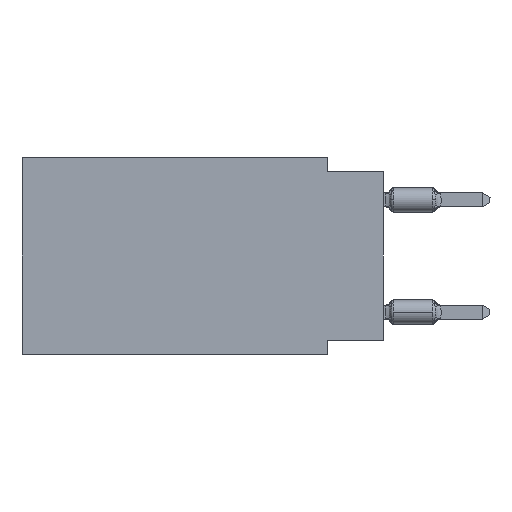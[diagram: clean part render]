
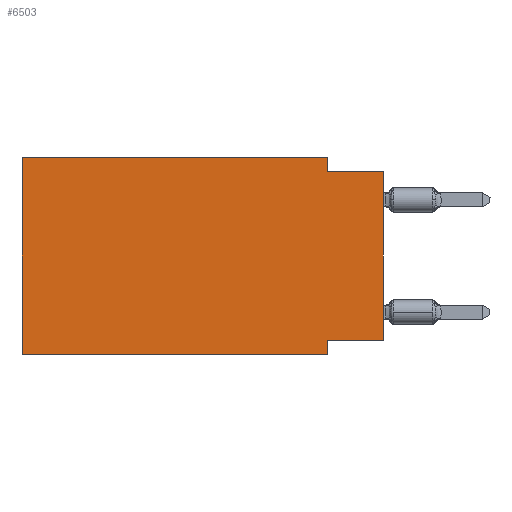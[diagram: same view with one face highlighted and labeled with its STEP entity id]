
A CAD part, left-side view. The second image highlights one B-rep face of the part: STEP entity #6503.
In plain terms, the highlighted planar face has unit normal (-1, 0, 0).
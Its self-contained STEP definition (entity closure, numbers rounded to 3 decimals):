
#836 = VECTOR ( 'NONE', #21411, 1000. ) ;
#2006 = DIRECTION ( 'NONE',  ( 0., -1., 0. ) ) ;
#2453 = CARTESIAN_POINT ( 'NONE',  ( 0., 0., -8.255 ) ) ;
#2573 = VERTEX_POINT ( 'NONE', #9083 ) ;
#2668 = ORIENTED_EDGE ( 'NONE', *, *, #27510, .F. ) ;
#3860 = VERTEX_POINT ( 'NONE', #21286 ) ;
#4321 = CARTESIAN_POINT ( 'NONE',  ( 0., 2.54, -0.635 ) ) ;
#4750 = CARTESIAN_POINT ( 'NONE',  ( 0., 2.54, -8.89 ) ) ;
#4767 = CARTESIAN_POINT ( 'NONE',  ( 0., 16.383, -8.89 ) ) ;
#6503 = ADVANCED_FACE ( 'NONE', ( #11510 ), #27806, .F. ) ;
#7463 = ORIENTED_EDGE ( 'NONE', *, *, #36338, .F. ) ;
#7663 = ORIENTED_EDGE ( 'NONE', *, *, #8486, .F. ) ;
#7884 = LINE ( 'NONE', #18130, #19427 ) ;
#8181 = LINE ( 'NONE', #14864, #32809 ) ;
#8486 = EDGE_CURVE ( 'NONE', #2573, #15020, #36292, .T. ) ;
#9083 = CARTESIAN_POINT ( 'NONE',  ( 0., 2.54, 0. ) ) ;
#10034 = EDGE_CURVE ( 'NONE', #3860, #40773, #40194, .T. ) ;
#10100 = VECTOR ( 'NONE', #2006, 1000. ) ;
#11232 = EDGE_LOOP ( 'NONE', ( #31197, #7463, #7663, #2668, #27136, #36452, #40490, #27331 ) ) ;
#11510 = FACE_OUTER_BOUND ( 'NONE', #11232, .T. ) ;
#11722 = CARTESIAN_POINT ( 'NONE',  ( 0., 16.383, 0. ) ) ;
#11844 = DIRECTION ( 'NONE',  ( 0., 0., 1. ) ) ;
#11952 = DIRECTION ( 'NONE',  ( 0., 0., -1. ) ) ;
#13986 = DIRECTION ( 'NONE',  ( 0., 0., 1. ) ) ;
#14433 = DIRECTION ( 'NONE',  ( 1., 0., 0. ) ) ;
#14538 = CARTESIAN_POINT ( 'NONE',  ( 0., 0., -0.635 ) ) ;
#14864 = CARTESIAN_POINT ( 'NONE',  ( 0., 16.383, 0. ) ) ;
#15020 = VERTEX_POINT ( 'NONE', #4321 ) ;
#18130 = CARTESIAN_POINT ( 'NONE',  ( 0., 16.383, 0. ) ) ;
#18974 = VECTOR ( 'NONE', #27931, 1000. ) ;
#19427 = VECTOR ( 'NONE', #11844, 1000. ) ;
#19973 = CARTESIAN_POINT ( 'NONE',  ( 0., 16.383, 0. ) ) ;
#21145 = DIRECTION ( 'NONE',  ( 0., -1., 0. ) ) ;
#21286 = CARTESIAN_POINT ( 'NONE',  ( 0., 2.54, -8.255 ) ) ;
#21411 = DIRECTION ( 'NONE',  ( 0., -1., 0. ) ) ;
#21619 = CARTESIAN_POINT ( 'NONE',  ( 0., 16.383, -8.89 ) ) ;
#22028 = AXIS2_PLACEMENT_3D ( 'NONE', #11722, #14433, #27381 ) ;
#22481 = EDGE_CURVE ( 'NONE', #31539, #40773, #31210, .T. ) ;
#26324 = LINE ( 'NONE', #26523, #29039 ) ;
#26523 = CARTESIAN_POINT ( 'NONE',  ( 0., 0., 0. ) ) ;
#27136 = ORIENTED_EDGE ( 'NONE', *, *, #33842, .F. ) ;
#27281 = VERTEX_POINT ( 'NONE', #29282 ) ;
#27331 = ORIENTED_EDGE ( 'NONE', *, *, #30565, .F. ) ;
#27381 = DIRECTION ( 'NONE',  ( 0., 0., -1. ) ) ;
#27510 = EDGE_CURVE ( 'NONE', #28054, #2573, #8181, .T. ) ;
#27806 = PLANE ( 'NONE',  #22028 ) ;
#27883 = VECTOR ( 'NONE', #11952, 1000. ) ;
#27931 = DIRECTION ( 'NONE',  ( 0., 1., 0. ) ) ;
#28054 = VERTEX_POINT ( 'NONE', #19973 ) ;
#29039 = VECTOR ( 'NONE', #13986, 1000. ) ;
#29282 = CARTESIAN_POINT ( 'NONE',  ( 0., 0., -8.255 ) ) ;
#29796 = DIRECTION ( 'NONE',  ( 0., 0., -1. ) ) ;
#30212 = LINE ( 'NONE', #14538, #10100 ) ;
#30565 = EDGE_CURVE ( 'NONE', #27281, #3860, #33797, .T. ) ;
#31197 = ORIENTED_EDGE ( 'NONE', *, *, #40412, .T. ) ;
#31210 = LINE ( 'NONE', #21619, #836 ) ;
#31539 = VERTEX_POINT ( 'NONE', #4767 ) ;
#31999 = VERTEX_POINT ( 'NONE', #40026 ) ;
#32113 = CARTESIAN_POINT ( 'NONE',  ( 0., 2.54, 0. ) ) ;
#32809 = VECTOR ( 'NONE', #21145, 1000. ) ;
#33797 = LINE ( 'NONE', #2453, #18974 ) ;
#33842 = EDGE_CURVE ( 'NONE', #31539, #28054, #7884, .T. ) ;
#36292 = LINE ( 'NONE', #32113, #37177 ) ;
#36338 = EDGE_CURVE ( 'NONE', #15020, #31999, #30212, .T. ) ;
#36452 = ORIENTED_EDGE ( 'NONE', *, *, #22481, .T. ) ;
#37177 = VECTOR ( 'NONE', #29796, 1000. ) ;
#40026 = CARTESIAN_POINT ( 'NONE',  ( 0., 0., -0.635 ) ) ;
#40194 = LINE ( 'NONE', #40611, #27883 ) ;
#40412 = EDGE_CURVE ( 'NONE', #27281, #31999, #26324, .T. ) ;
#40490 = ORIENTED_EDGE ( 'NONE', *, *, #10034, .F. ) ;
#40611 = CARTESIAN_POINT ( 'NONE',  ( 0., 2.54, -8.89 ) ) ;
#40773 = VERTEX_POINT ( 'NONE', #4750 ) ;
